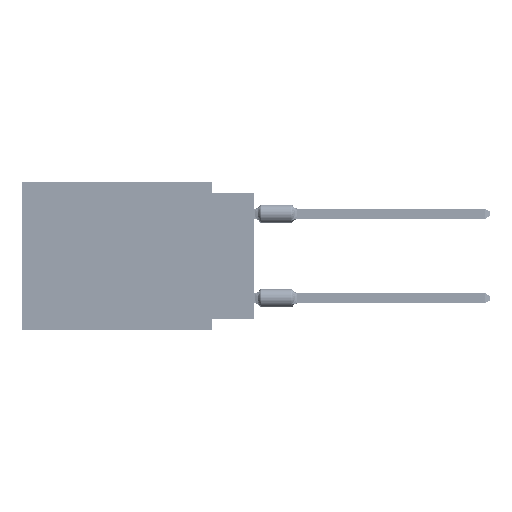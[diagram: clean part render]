
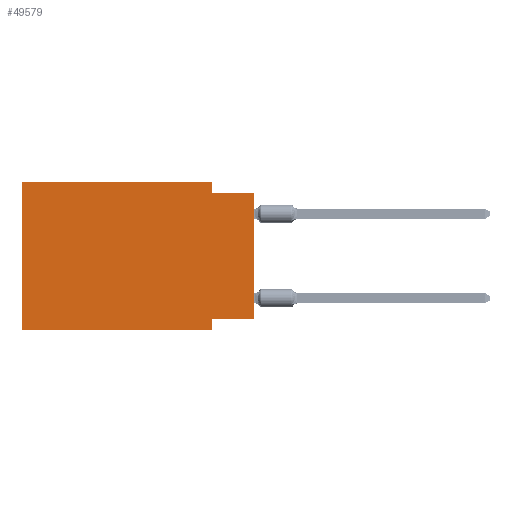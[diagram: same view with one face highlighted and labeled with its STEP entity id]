
A CAD part, left-side view. The second image highlights one B-rep face of the part: STEP entity #49579.
In plain terms, the highlighted planar face has unit normal (-1, 0, 0).
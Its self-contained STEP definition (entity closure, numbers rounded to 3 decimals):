
#2413 = VERTEX_POINT ( 'NONE', #70925 ) ;
#2947 = DIRECTION ( 'NONE',  ( 0., 0., 1. ) ) ;
#3914 = VERTEX_POINT ( 'NONE', #33290 ) ;
#5224 = VECTOR ( 'NONE', #55797, 1000. ) ;
#5352 = CARTESIAN_POINT ( 'NONE',  ( 0., 13.97, 0. ) ) ;
#6144 = CARTESIAN_POINT ( 'NONE',  ( 0., 0., -0.635 ) ) ;
#6240 = EDGE_CURVE ( 'NONE', #71662, #103691, #39385, .T. ) ;
#6399 = VECTOR ( 'NONE', #93843, 1000. ) ;
#7464 = CARTESIAN_POINT ( 'NONE',  ( 0., 0., -8.255 ) ) ;
#9650 = VERTEX_POINT ( 'NONE', #53756 ) ;
#10639 = ORIENTED_EDGE ( 'NONE', *, *, #54289, .T. ) ;
#11626 = VERTEX_POINT ( 'NONE', #83769 ) ;
#14509 = CARTESIAN_POINT ( 'NONE',  ( 0., 2.54, -8.89 ) ) ;
#16535 = VECTOR ( 'NONE', #89299, 1000. ) ;
#16730 = LINE ( 'NONE', #71331, #16535 ) ;
#20256 = ORIENTED_EDGE ( 'NONE', *, *, #21281, .F. ) ;
#21281 = EDGE_CURVE ( 'NONE', #3914, #11626, #102279, .T. ) ;
#21522 = CARTESIAN_POINT ( 'NONE',  ( 0., 2.54, -8.89 ) ) ;
#22210 = VECTOR ( 'NONE', #79750, 1000. ) ;
#22391 = EDGE_CURVE ( 'NONE', #78704, #71662, #80030, .T. ) ;
#29204 = DIRECTION ( 'NONE',  ( 0., -1., 0. ) ) ;
#29716 = CARTESIAN_POINT ( 'NONE',  ( 0., 2.54, 0. ) ) ;
#29744 = ORIENTED_EDGE ( 'NONE', *, *, #97591, .T. ) ;
#30312 = CARTESIAN_POINT ( 'NONE',  ( 0., 0., -8.255 ) ) ;
#32836 = ORIENTED_EDGE ( 'NONE', *, *, #54413, .F. ) ;
#33290 = CARTESIAN_POINT ( 'NONE',  ( 0., 2.54, 0. ) ) ;
#35569 = ORIENTED_EDGE ( 'NONE', *, *, #6240, .F. ) ;
#39385 = LINE ( 'NONE', #14509, #5224 ) ;
#39824 = EDGE_CURVE ( 'NONE', #2413, #3914, #75336, .T. ) ;
#40938 = EDGE_CURVE ( 'NONE', #11626, #9650, #94087, .T. ) ;
#42087 = FACE_OUTER_BOUND ( 'NONE', #54770, .T. ) ;
#42631 = DIRECTION ( 'NONE',  ( 0., 0., -1. ) ) ;
#46890 = AXIS2_PLACEMENT_3D ( 'NONE', #99309, #50574, #42631 ) ;
#47141 = CARTESIAN_POINT ( 'NONE',  ( 0., 13.97, -8.89 ) ) ;
#49579 = ADVANCED_FACE ( 'NONE', ( #42087 ), #66503, .F. ) ;
#50574 = DIRECTION ( 'NONE',  ( 1., 0., 0. ) ) ;
#53035 = ORIENTED_EDGE ( 'NONE', *, *, #22391, .F. ) ;
#53632 = CARTESIAN_POINT ( 'NONE',  ( 0., 0., 0. ) ) ;
#53756 = CARTESIAN_POINT ( 'NONE',  ( 0., 0., -0.635 ) ) ;
#54289 = EDGE_CURVE ( 'NONE', #57660, #103691, #16730, .T. ) ;
#54413 = EDGE_CURVE ( 'NONE', #57660, #2413, #98838, .T. ) ;
#54770 = EDGE_LOOP ( 'NONE', ( #29744, #88032, #20256, #89216, #32836, #10639, #35569, #53035 ) ) ;
#55797 = DIRECTION ( 'NONE',  ( 0., 0., -1. ) ) ;
#57377 = VECTOR ( 'NONE', #29204, 1000. ) ;
#57660 = VERTEX_POINT ( 'NONE', #47141 ) ;
#58066 = CARTESIAN_POINT ( 'NONE',  ( 0., 13.97, 0. ) ) ;
#61083 = CARTESIAN_POINT ( 'NONE',  ( 0., 2.54, -8.255 ) ) ;
#66503 = PLANE ( 'NONE',  #46890 ) ;
#67150 = VECTOR ( 'NONE', #78949, 1000. ) ;
#68511 = DIRECTION ( 'NONE',  ( 0., 0., 1. ) ) ;
#70925 = CARTESIAN_POINT ( 'NONE',  ( 0., 13.97, 0. ) ) ;
#71331 = CARTESIAN_POINT ( 'NONE',  ( 0., 13.97, -8.89 ) ) ;
#71662 = VERTEX_POINT ( 'NONE', #61083 ) ;
#75336 = LINE ( 'NONE', #5352, #57377 ) ;
#78704 = VERTEX_POINT ( 'NONE', #30312 ) ;
#78949 = DIRECTION ( 'NONE',  ( 0., 0., -1. ) ) ;
#79750 = DIRECTION ( 'NONE',  ( 0., -1., 0. ) ) ;
#80030 = LINE ( 'NONE', #7464, #6399 ) ;
#83769 = CARTESIAN_POINT ( 'NONE',  ( 0., 2.54, -0.635 ) ) ;
#84205 = VECTOR ( 'NONE', #2947, 1000. ) ;
#88032 = ORIENTED_EDGE ( 'NONE', *, *, #40938, .F. ) ;
#89216 = ORIENTED_EDGE ( 'NONE', *, *, #39824, .F. ) ;
#89299 = DIRECTION ( 'NONE',  ( 0., -1., 0. ) ) ;
#90932 = VECTOR ( 'NONE', #68511, 1000. ) ;
#93843 = DIRECTION ( 'NONE',  ( 0., 1., 0. ) ) ;
#94087 = LINE ( 'NONE', #6144, #22210 ) ;
#97591 = EDGE_CURVE ( 'NONE', #78704, #9650, #101310, .T. ) ;
#98838 = LINE ( 'NONE', #58066, #84205 ) ;
#99309 = CARTESIAN_POINT ( 'NONE',  ( 0., 13.97, 0. ) ) ;
#101310 = LINE ( 'NONE', #53632, #90932 ) ;
#102279 = LINE ( 'NONE', #29716, #67150 ) ;
#103691 = VERTEX_POINT ( 'NONE', #21522 ) ;
